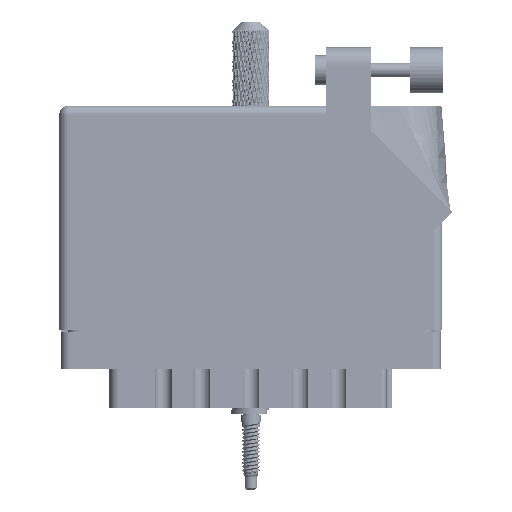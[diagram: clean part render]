
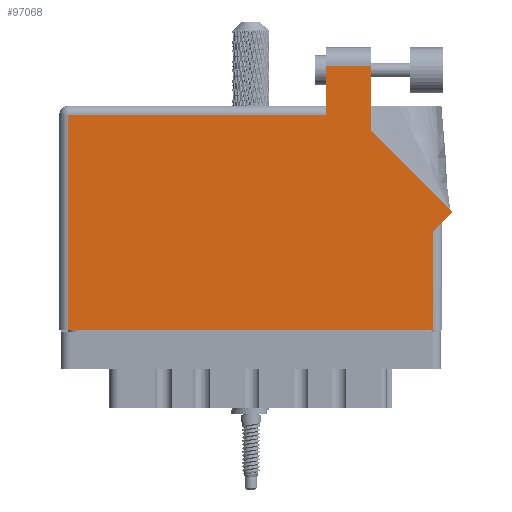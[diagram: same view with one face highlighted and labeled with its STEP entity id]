
A CAD part, front view. The second image highlights one B-rep face of the part: STEP entity #97068.
In plain terms, the highlighted face is planar.
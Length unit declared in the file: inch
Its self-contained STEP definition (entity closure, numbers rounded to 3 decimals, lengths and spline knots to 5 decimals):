
#4380 = ORIENTED_EDGE ( 'NONE', *, *, #38163, .T. ) ;
#4790 = EDGE_LOOP ( 'NONE', ( #91222, #43703, #63409, #118828, #25014, #80822, #37785, #4380, #20556 ) ) ;
#7004 = CARTESIAN_POINT ( 'NONE',  ( 2.55, 0.737, 0. ) ) ;
#8666 = VECTOR ( 'NONE', #92314, 39.37008 ) ;
#10036 = VECTOR ( 'NONE', #32035, 39.37008 ) ;
#11402 = EDGE_CURVE ( 'NONE', #28376, #110424, #37037, .T. ) ;
#12229 = DIRECTION ( 'NONE',  ( 1., 0., 0. ) ) ;
#12527 = CARTESIAN_POINT ( 'NONE',  ( 1.819, 1.53, 0. ) ) ;
#16918 = LINE ( 'NONE', #108595, #67404 ) ;
#20204 = LINE ( 'NONE', #7004, #115431 ) ;
#20556 = ORIENTED_EDGE ( 'NONE', *, *, #76722, .T. ) ;
#21531 = VERTEX_POINT ( 'NONE', #111408 ) ;
#23642 = VECTOR ( 'NONE', #41674, 39.37008 ) ;
#23877 = CARTESIAN_POINT ( 'NONE',  ( 2.68271, 0.80771, 0. ) ) ;
#24440 = EDGE_CURVE ( 'NONE', #21531, #89182, #67294, .T. ) ;
#25014 = ORIENTED_EDGE ( 'NONE', *, *, #31736, .T. ) ;
#28376 = VERTEX_POINT ( 'NONE', #90908 ) ;
#31730 = LINE ( 'NONE', #36345, #8666 ) ;
#31736 = EDGE_CURVE ( 'NONE', #87642, #21531, #56879, .T. ) ;
#32035 = DIRECTION ( 'NONE',  ( -0.707, 0.707, 0. ) ) ;
#34563 = VECTOR ( 'NONE', #78862, 39.37008 ) ;
#36345 = CARTESIAN_POINT ( 'NONE',  ( 1.819, 1.805, 0. ) ) ;
#37037 = LINE ( 'NONE', #67297, #39945 ) ;
#37785 = ORIENTED_EDGE ( 'NONE', *, *, #106515, .T. ) ;
#38163 = EDGE_CURVE ( 'NONE', #84509, #55770, #96533, .T. ) ;
#39945 = VECTOR ( 'NONE', #67000, 39.37008 ) ;
#41674 = DIRECTION ( 'NONE',  ( 0., -1., 0. ) ) ;
#43703 = ORIENTED_EDGE ( 'NONE', *, *, #115040, .T. ) ;
#44143 = DIRECTION ( 'NONE',  ( -1., 0., 0. ) ) ;
#47997 = CARTESIAN_POINT ( 'NONE',  ( 2.55, 0.675, 0. ) ) ;
#49297 = DIRECTION ( 'NONE',  ( 0., -1., 0. ) ) ;
#55770 = VERTEX_POINT ( 'NONE', #23877 ) ;
#56879 = LINE ( 'NONE', #97984, #23642 ) ;
#57392 = CARTESIAN_POINT ( 'NONE',  ( 0., 0., 0. ) ) ;
#59384 = VERTEX_POINT ( 'NONE', #85505 ) ;
#60336 = CARTESIAN_POINT ( 'NONE',  ( 2.612, 0.737, 0. ) ) ;
#62094 = FACE_OUTER_BOUND ( 'NONE', #4790, .T. ) ;
#63409 = ORIENTED_EDGE ( 'NONE', *, *, #63853, .T. ) ;
#63853 = EDGE_CURVE ( 'NONE', #59384, #67775, #100532, .T. ) ;
#67000 = DIRECTION ( 'NONE',  ( 0., 1., 0. ) ) ;
#67294 = LINE ( 'NONE', #57392, #108966 ) ;
#67297 = CARTESIAN_POINT ( 'NONE',  ( 2.126, 1.36442, 0. ) ) ;
#67404 = VECTOR ( 'NONE', #92012, 39.37008 ) ;
#67775 = VERTEX_POINT ( 'NONE', #86391 ) ;
#72349 = DIRECTION ( 'NONE',  ( 0., 0., -1. ) ) ;
#73157 = CARTESIAN_POINT ( 'NONE',  ( 0., 1.53, 0. ) ) ;
#76722 = EDGE_CURVE ( 'NONE', #55770, #28376, #105187, .T. ) ;
#78862 = DIRECTION ( 'NONE',  ( 0.707, 0.707, 0. ) ) ;
#80744 = EDGE_CURVE ( 'NONE', #67775, #87642, #16918, .T. ) ;
#80822 = ORIENTED_EDGE ( 'NONE', *, *, #24440, .T. ) ;
#84509 = VERTEX_POINT ( 'NONE', #47997 ) ;
#85505 = CARTESIAN_POINT ( 'NONE',  ( 1.819, 1.805, 0. ) ) ;
#86391 = CARTESIAN_POINT ( 'NONE',  ( 1.819, 1.468, 0. ) ) ;
#86897 = CARTESIAN_POINT ( 'NONE',  ( 2.68271, 0.80771, 0. ) ) ;
#87642 = VERTEX_POINT ( 'NONE', #91411 ) ;
#89182 = VERTEX_POINT ( 'NONE', #98088 ) ;
#90908 = CARTESIAN_POINT ( 'NONE',  ( 2.126, 1.36442, 0. ) ) ;
#91222 = ORIENTED_EDGE ( 'NONE', *, *, #11402, .T. ) ;
#91411 = CARTESIAN_POINT ( 'NONE',  ( 0.062, 1.468, 0. ) ) ;
#92012 = DIRECTION ( 'NONE',  ( -1., 0., 0. ) ) ;
#92314 = DIRECTION ( 'NONE',  ( -1., 0., 0. ) ) ;
#92675 = CARTESIAN_POINT ( 'NONE',  ( 2.126, 1.805, 0. ) ) ;
#96533 = LINE ( 'NONE', #60336, #34563 ) ;
#97068 = ADVANCED_FACE ( 'NONE', ( #62094 ), #99265, .F. ) ;
#97984 = CARTESIAN_POINT ( 'NONE',  ( 0.062, 0., 0. ) ) ;
#98088 = CARTESIAN_POINT ( 'NONE',  ( 2.55, 0., 0. ) ) ;
#98848 = DIRECTION ( 'NONE',  ( 0., 1., 0. ) ) ;
#99265 = PLANE ( 'NONE',  #100903 ) ;
#100532 = LINE ( 'NONE', #12527, #101927 ) ;
#100903 = AXIS2_PLACEMENT_3D ( 'NONE', #73157, #72349, #44143 ) ;
#101927 = VECTOR ( 'NONE', #49297, 39.37008 ) ;
#105187 = LINE ( 'NONE', #86897, #10036 ) ;
#106515 = EDGE_CURVE ( 'NONE', #89182, #84509, #20204, .T. ) ;
#108595 = CARTESIAN_POINT ( 'NONE',  ( 0., 1.468, 0. ) ) ;
#108966 = VECTOR ( 'NONE', #12229, 39.37008 ) ;
#110424 = VERTEX_POINT ( 'NONE', #92675 ) ;
#111408 = CARTESIAN_POINT ( 'NONE',  ( 0.062, 0., 0. ) ) ;
#115040 = EDGE_CURVE ( 'NONE', #110424, #59384, #31730, .T. ) ;
#115431 = VECTOR ( 'NONE', #98848, 39.37008 ) ;
#118828 = ORIENTED_EDGE ( 'NONE', *, *, #80744, .T. ) ;
